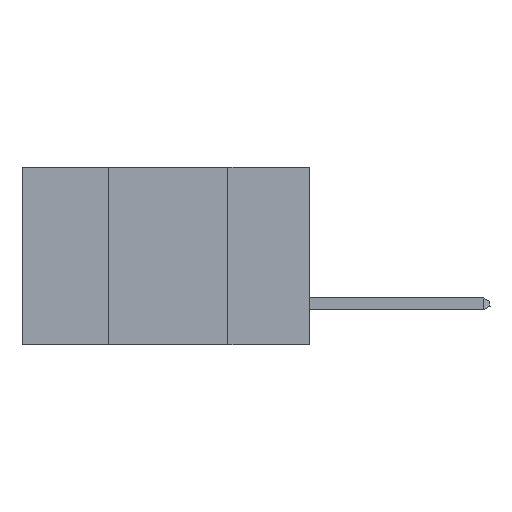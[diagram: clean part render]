
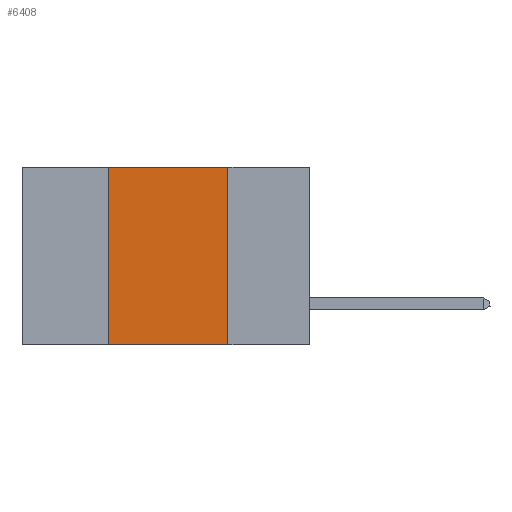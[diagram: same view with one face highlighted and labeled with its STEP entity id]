
A CAD part, left-side view. The second image highlights one B-rep face of the part: STEP entity #6408.
In plain terms, the highlighted planar face has unit normal (-1, 0, 0).
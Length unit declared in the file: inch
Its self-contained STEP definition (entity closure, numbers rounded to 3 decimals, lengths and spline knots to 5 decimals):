
#1224 = DIRECTION ( 'NONE',  ( 0., -1., 0. ) ) ;
#2494 = CARTESIAN_POINT ( 'NONE',  ( 0., 0.42, -0.37 ) ) ;
#3317 = LINE ( 'NONE', #8897, #13697 ) ;
#3385 = DIRECTION ( 'NONE',  ( 0., 0., -1. ) ) ;
#3783 = CARTESIAN_POINT ( 'NONE',  ( 0., 0.17, 0. ) ) ;
#4456 = VERTEX_POINT ( 'NONE', #2494 ) ;
#4574 = EDGE_CURVE ( 'NONE', #4456, #16765, #9831, .T. ) ;
#4788 = ORIENTED_EDGE ( 'NONE', *, *, #15394, .F. ) ;
#5099 = CARTESIAN_POINT ( 'NONE',  ( 0., 0.6, 0. ) ) ;
#5597 = EDGE_CURVE ( 'NONE', #4456, #15366, #3317, .T. ) ;
#5815 = VECTOR ( 'NONE', #10635, 39.37008 ) ;
#5957 = CARTESIAN_POINT ( 'NONE',  ( 0., 0.17, 0. ) ) ;
#6182 = DIRECTION ( 'NONE',  ( 0., 0., -1. ) ) ;
#6345 = VERTEX_POINT ( 'NONE', #3783 ) ;
#6408 = ADVANCED_FACE ( 'NONE', ( #10987 ), #8670, .F. ) ;
#7662 = DIRECTION ( 'NONE',  ( 0., -1., 0. ) ) ;
#8571 = CARTESIAN_POINT ( 'NONE',  ( 0., 0.42, 0. ) ) ;
#8670 = PLANE ( 'NONE',  #10135 ) ;
#8692 = VECTOR ( 'NONE', #1224, 39.37008 ) ;
#8897 = CARTESIAN_POINT ( 'NONE',  ( 0., 0.6, -0.37 ) ) ;
#9372 = ORIENTED_EDGE ( 'NONE', *, *, #13104, .F. ) ;
#9831 = LINE ( 'NONE', #15932, #5815 ) ;
#10135 = AXIS2_PLACEMENT_3D ( 'NONE', #16561, #13975, #6182 ) ;
#10635 = DIRECTION ( 'NONE',  ( 0., 0., 1. ) ) ;
#10636 = ORIENTED_EDGE ( 'NONE', *, *, #5597, .T. ) ;
#10987 = FACE_OUTER_BOUND ( 'NONE', #11850, .T. ) ;
#11850 = EDGE_LOOP ( 'NONE', ( #4788, #9372, #16776, #10636 ) ) ;
#12001 = LINE ( 'NONE', #5957, #14066 ) ;
#12560 = LINE ( 'NONE', #5099, #8692 ) ;
#13104 = EDGE_CURVE ( 'NONE', #16765, #6345, #12560, .T. ) ;
#13528 = CARTESIAN_POINT ( 'NONE',  ( 0., 0.17, -0.37 ) ) ;
#13697 = VECTOR ( 'NONE', #7662, 39.37008 ) ;
#13975 = DIRECTION ( 'NONE',  ( 1., 0., 0. ) ) ;
#14066 = VECTOR ( 'NONE', #3385, 39.37008 ) ;
#15366 = VERTEX_POINT ( 'NONE', #13528 ) ;
#15394 = EDGE_CURVE ( 'NONE', #6345, #15366, #12001, .T. ) ;
#15932 = CARTESIAN_POINT ( 'NONE',  ( 0., 0.42, 0. ) ) ;
#16561 = CARTESIAN_POINT ( 'NONE',  ( 0., 0.6, 0. ) ) ;
#16765 = VERTEX_POINT ( 'NONE', #8571 ) ;
#16776 = ORIENTED_EDGE ( 'NONE', *, *, #4574, .F. ) ;
